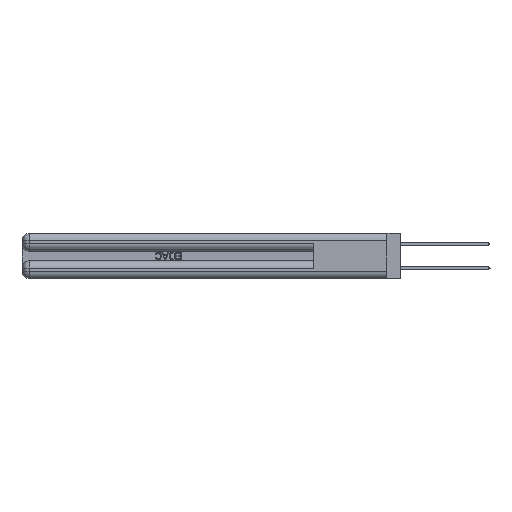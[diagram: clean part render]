
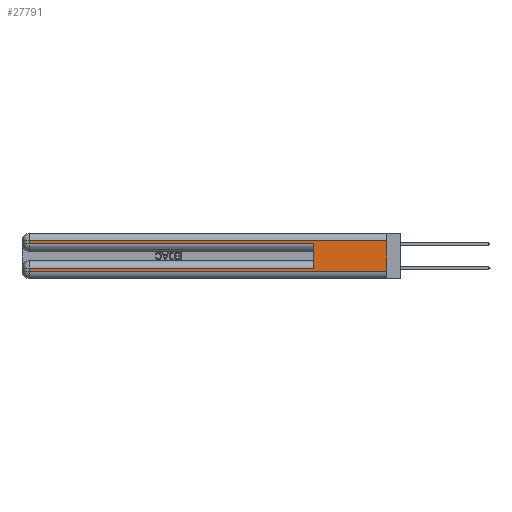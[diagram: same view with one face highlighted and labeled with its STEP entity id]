
A CAD part, left-side view. The second image highlights one B-rep face of the part: STEP entity #27791.
In plain terms, the highlighted planar face has unit normal (-1, 0, 0).
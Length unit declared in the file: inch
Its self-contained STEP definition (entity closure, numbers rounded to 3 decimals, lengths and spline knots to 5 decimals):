
#296 = DIRECTION ( 'NONE',  ( 0., 0., -1. ) ) ;
#751 = CARTESIAN_POINT ( 'NONE',  ( 0., 0., 0.06 ) ) ;
#1170 = DIRECTION ( 'NONE',  ( 0., 1., 0. ) ) ;
#3218 = LINE ( 'NONE', #9219, #30912 ) ;
#4261 = LINE ( 'NONE', #5129, #10493 ) ;
#5032 = VECTOR ( 'NONE', #1170, 39.37008 ) ;
#5129 = CARTESIAN_POINT ( 'NONE',  ( 0., 0., 0.085 ) ) ;
#5329 = ORIENTED_EDGE ( 'NONE', *, *, #6825, .T. ) ;
#6825 = EDGE_CURVE ( 'NONE', #31633, #37403, #3218, .T. ) ;
#6979 = VERTEX_POINT ( 'NONE', #41312 ) ;
#7436 = EDGE_CURVE ( 'NONE', #45954, #31633, #4261, .T. ) ;
#8816 = AXIS2_PLACEMENT_3D ( 'NONE', #18276, #43456, #296 ) ;
#9219 = CARTESIAN_POINT ( 'NONE',  ( 0., 2.94, 0.37 ) ) ;
#10301 = VERTEX_POINT ( 'NONE', #22130 ) ;
#10493 = VECTOR ( 'NONE', #12052, 39.37008 ) ;
#10783 = VECTOR ( 'NONE', #16771, 39.37008 ) ;
#11437 = EDGE_CURVE ( 'NONE', #6979, #10301, #16708, .T. ) ;
#11449 = CARTESIAN_POINT ( 'NONE',  ( 0., 0.6, 0.285 ) ) ;
#12052 = DIRECTION ( 'NONE',  ( 0., 1., 0. ) ) ;
#12213 = VECTOR ( 'NONE', #36628, 39.37008 ) ;
#12783 = ORIENTED_EDGE ( 'NONE', *, *, #27347, .F. ) ;
#15542 = ORIENTED_EDGE ( 'NONE', *, *, #45934, .T. ) ;
#16481 = DIRECTION ( 'NONE',  ( 0., 0., 1. ) ) ;
#16708 = LINE ( 'NONE', #32024, #42746 ) ;
#16771 = DIRECTION ( 'NONE',  ( 0., 0., -1. ) ) ;
#16919 = CARTESIAN_POINT ( 'NONE',  ( 0., 0., 0.37 ) ) ;
#17124 = LINE ( 'NONE', #751, #30172 ) ;
#18276 = CARTESIAN_POINT ( 'NONE',  ( 0., 0., 0.37 ) ) ;
#18668 = CARTESIAN_POINT ( 'NONE',  ( 0., 0., 0.31 ) ) ;
#19102 = CARTESIAN_POINT ( 'NONE',  ( 0., 0., 0.31 ) ) ;
#21001 = EDGE_CURVE ( 'NONE', #37403, #33959, #17124, .T. ) ;
#21781 = LINE ( 'NONE', #32974, #12213 ) ;
#21812 = DIRECTION ( 'NONE',  ( 0., 0., -1. ) ) ;
#22130 = CARTESIAN_POINT ( 'NONE',  ( 0., 2.94, 0.285 ) ) ;
#24246 = ORIENTED_EDGE ( 'NONE', *, *, #30418, .F. ) ;
#25531 = DIRECTION ( 'NONE',  ( 0., -1., 0. ) ) ;
#26132 = EDGE_LOOP ( 'NONE', ( #24246, #39086, #36796, #15542, #12783, #38950, #5329, #41374 ) ) ;
#27347 = EDGE_CURVE ( 'NONE', #45954, #37137, #35299, .T. ) ;
#27579 = CARTESIAN_POINT ( 'NONE',  ( 0., 2.94, 0.06 ) ) ;
#27791 = ADVANCED_FACE ( 'NONE', ( #44261 ), #29384, .F. ) ;
#29384 = PLANE ( 'NONE',  #8816 ) ;
#30172 = VECTOR ( 'NONE', #25531, 39.37008 ) ;
#30418 = EDGE_CURVE ( 'NONE', #43945, #33959, #41360, .T. ) ;
#30912 = VECTOR ( 'NONE', #41328, 39.37008 ) ;
#31633 = VERTEX_POINT ( 'NONE', #34953 ) ;
#32024 = CARTESIAN_POINT ( 'NONE',  ( 0., 2.94, 0.37 ) ) ;
#32974 = CARTESIAN_POINT ( 'NONE',  ( 0., 0., 0.285 ) ) ;
#33959 = VERTEX_POINT ( 'NONE', #46582 ) ;
#34045 = CARTESIAN_POINT ( 'NONE',  ( 0., 0.6, 0.145 ) ) ;
#34953 = CARTESIAN_POINT ( 'NONE',  ( 0., 2.94, 0.085 ) ) ;
#35299 = LINE ( 'NONE', #34045, #36941 ) ;
#36628 = DIRECTION ( 'NONE',  ( 0., -1., 0. ) ) ;
#36796 = ORIENTED_EDGE ( 'NONE', *, *, #11437, .T. ) ;
#36941 = VECTOR ( 'NONE', #16481, 39.37008 ) ;
#37137 = VERTEX_POINT ( 'NONE', #11449 ) ;
#37403 = VERTEX_POINT ( 'NONE', #27579 ) ;
#38950 = ORIENTED_EDGE ( 'NONE', *, *, #7436, .T. ) ;
#39086 = ORIENTED_EDGE ( 'NONE', *, *, #44890, .T. ) ;
#39922 = CARTESIAN_POINT ( 'NONE',  ( 0., 0.6, 0.085 ) ) ;
#41312 = CARTESIAN_POINT ( 'NONE',  ( 0., 2.94, 0.31 ) ) ;
#41328 = DIRECTION ( 'NONE',  ( 0., 0., -1. ) ) ;
#41360 = LINE ( 'NONE', #16919, #10783 ) ;
#41374 = ORIENTED_EDGE ( 'NONE', *, *, #21001, .T. ) ;
#42746 = VECTOR ( 'NONE', #21812, 39.37008 ) ;
#43456 = DIRECTION ( 'NONE',  ( 1., 0., 0. ) ) ;
#43945 = VERTEX_POINT ( 'NONE', #18668 ) ;
#44261 = FACE_OUTER_BOUND ( 'NONE', #26132, .T. ) ;
#44573 = LINE ( 'NONE', #19102, #5032 ) ;
#44890 = EDGE_CURVE ( 'NONE', #43945, #6979, #44573, .T. ) ;
#45934 = EDGE_CURVE ( 'NONE', #10301, #37137, #21781, .T. ) ;
#45954 = VERTEX_POINT ( 'NONE', #39922 ) ;
#46582 = CARTESIAN_POINT ( 'NONE',  ( 0., 0., 0.06 ) ) ;
